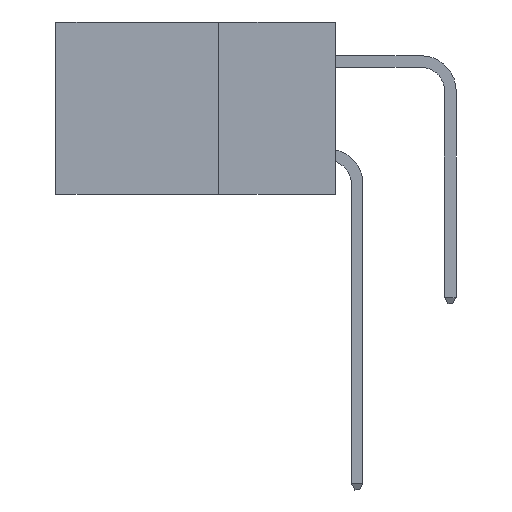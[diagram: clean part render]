
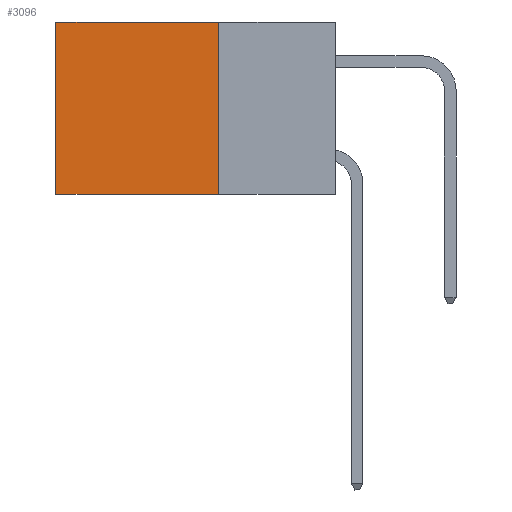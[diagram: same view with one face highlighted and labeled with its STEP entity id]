
A CAD part, left-side view. The second image highlights one B-rep face of the part: STEP entity #3096.
In plain terms, the highlighted planar face has unit normal (-1, 0, 0).
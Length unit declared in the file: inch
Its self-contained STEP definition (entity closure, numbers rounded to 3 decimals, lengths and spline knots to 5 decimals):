
#24 = DIRECTION ( 'NONE',  ( 0., 0., -1. ) ) ;
#132 = LINE ( 'NONE', #24531, #19143 ) ;
#1381 = DIRECTION ( 'NONE',  ( 0., 0., -1. ) ) ;
#2471 = LINE ( 'NONE', #7049, #26389 ) ;
#3087 = CARTESIAN_POINT ( 'NONE',  ( 0.2875, 0.25, 0. ) ) ;
#3096 = ADVANCED_FACE ( 'NONE', ( #5368 ), #7660, .F. ) ;
#3818 = CARTESIAN_POINT ( 'NONE',  ( 0.2875, 0.6, 0. ) ) ;
#4673 = ORIENTED_EDGE ( 'NONE', *, *, #21246, .T. ) ;
#4987 = LINE ( 'NONE', #11631, #11445 ) ;
#5368 = FACE_OUTER_BOUND ( 'NONE', #13231, .T. ) ;
#5799 = DIRECTION ( 'NONE',  ( 0., 0., -1. ) ) ;
#6101 = ORIENTED_EDGE ( 'NONE', *, *, #11918, .F. ) ;
#6354 = VECTOR ( 'NONE', #1381, 39.37008 ) ;
#7049 = CARTESIAN_POINT ( 'NONE',  ( 0.2875, 0.25, 0. ) ) ;
#7660 = PLANE ( 'NONE',  #12973 ) ;
#8292 = CARTESIAN_POINT ( 'NONE',  ( 0.2875, 0.6, -0.37 ) ) ;
#8834 = ORIENTED_EDGE ( 'NONE', *, *, #27387, .T. ) ;
#9207 = CARTESIAN_POINT ( 'NONE',  ( 0.2875, 0.6, 0. ) ) ;
#10799 = DIRECTION ( 'NONE',  ( 0., 1., 0. ) ) ;
#11445 = VECTOR ( 'NONE', #16409, 39.37008 ) ;
#11631 = CARTESIAN_POINT ( 'NONE',  ( 0.2875, 0.25, -0.37 ) ) ;
#11918 = EDGE_CURVE ( 'NONE', #14449, #16571, #2471, .T. ) ;
#12973 = AXIS2_PLACEMENT_3D ( 'NONE', #3087, #27366, #5799 ) ;
#13231 = EDGE_LOOP ( 'NONE', ( #4673, #26873, #6101, #8834 ) ) ;
#14449 = VERTEX_POINT ( 'NONE', #28399 ) ;
#16409 = DIRECTION ( 'NONE',  ( 0., 1., 0. ) ) ;
#16571 = VERTEX_POINT ( 'NONE', #22402 ) ;
#18359 = VERTEX_POINT ( 'NONE', #9207 ) ;
#19143 = VECTOR ( 'NONE', #10799, 39.37008 ) ;
#19414 = VERTEX_POINT ( 'NONE', #8292 ) ;
#21246 = EDGE_CURVE ( 'NONE', #18359, #19414, #27986, .T. ) ;
#22402 = CARTESIAN_POINT ( 'NONE',  ( 0.2875, 0.25, -0.37 ) ) ;
#22469 = EDGE_CURVE ( 'NONE', #16571, #19414, #4987, .T. ) ;
#24531 = CARTESIAN_POINT ( 'NONE',  ( 0.2875, 0.25, 0. ) ) ;
#26389 = VECTOR ( 'NONE', #24, 39.37008 ) ;
#26873 = ORIENTED_EDGE ( 'NONE', *, *, #22469, .F. ) ;
#27366 = DIRECTION ( 'NONE',  ( 1., 0., 0. ) ) ;
#27387 = EDGE_CURVE ( 'NONE', #14449, #18359, #132, .T. ) ;
#27986 = LINE ( 'NONE', #3818, #6354 ) ;
#28399 = CARTESIAN_POINT ( 'NONE',  ( 0.2875, 0.25, 0. ) ) ;
